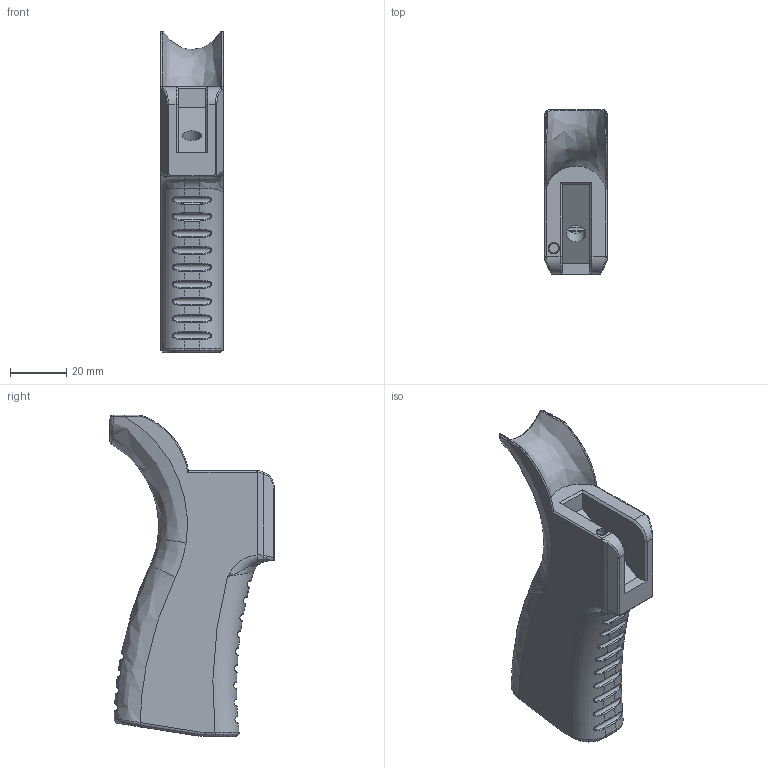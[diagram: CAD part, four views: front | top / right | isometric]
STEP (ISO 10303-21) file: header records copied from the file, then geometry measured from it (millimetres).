
FILE_DESCRIPTION(/* description */ (''),/* implementation_level */ '2;1');
FILE_NAME(/* name */ 'Grip 1.step',/* time_stamp */ '2021-10-28T08:42:24-04:00',/* author */ (''),/* organization */ (''),/* preprocessor_version */ 'ST-DEVELOPER v18.1',/* originating_system */ 'Autodesk Translation Framework v10.10.0.1391',/* authorisation */ '');
FILE_SCHEMA (('AUTOMOTIVE_DESIGN { 1 0 10303 214 3 1 1 }'));
Products named in the file (1): Grip 1
Bounding box: 22.33 x 58.4 x 113.9 mm (x, y, z)
Volume: 47326 mm3; surface area: 21615 mm2
Topology: 1 solids, 1 shells, 770 faces, 2030 edges, 1206 vertices
Faces by surface type: bspline 491, cylinder 142, plane 69, torus 57, cone 9, sphere 2
Full cylindrical faces by diameter (mm): 3.4 x1, 6.8 x1, 11.616 x1, 13.416 x1
Entity records: 40041 total; most frequent: CARTESIAN_POINT 24277, ORIENTED_EDGE 3920, DIRECTION 2220, EDGE_CURVE 1960, VERTEX_POINT 1206, B_SPLINE_CURVE_WITH_KNOTS 833, AXIS2_PLACEMENT_3D 814, EDGE_LOOP 786
